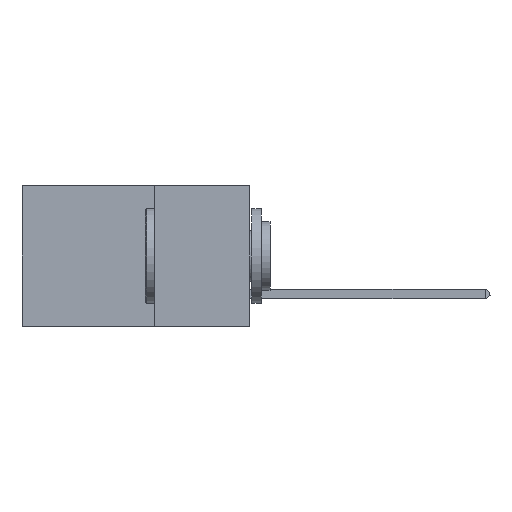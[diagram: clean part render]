
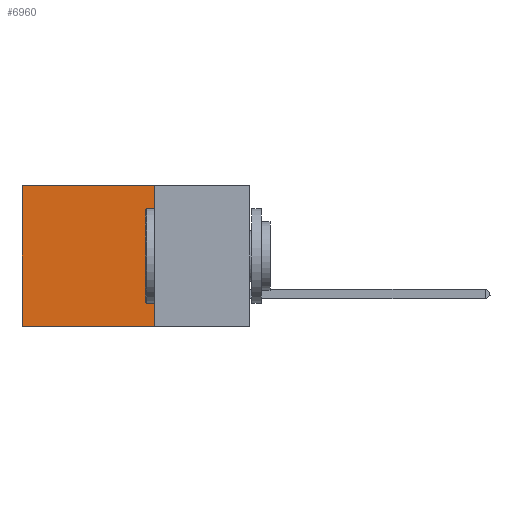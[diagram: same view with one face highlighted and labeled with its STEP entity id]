
A CAD part, left-side view. The second image highlights one B-rep face of the part: STEP entity #6960.
In plain terms, the highlighted planar face has unit normal (-1, 0, 0).
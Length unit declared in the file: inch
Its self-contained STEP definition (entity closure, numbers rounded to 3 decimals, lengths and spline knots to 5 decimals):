
#1176 = ORIENTED_EDGE ( 'NONE', *, *, #7756, .F. ) ;
#1188 = DIRECTION ( 'NONE',  ( 0., 0., -1. ) ) ;
#2180 = DIRECTION ( 'NONE',  ( 0., 1., 0. ) ) ;
#2406 = DIRECTION ( 'NONE',  ( 0., 0., -1. ) ) ;
#2745 = VECTOR ( 'NONE', #12073, 39.37008 ) ;
#2907 = CARTESIAN_POINT ( 'NONE',  ( 0.2875, 0.25, -0.37 ) ) ;
#2998 = VERTEX_POINT ( 'NONE', #14916 ) ;
#4323 = EDGE_CURVE ( 'NONE', #6081, #2998, #13148, .T. ) ;
#4479 = EDGE_CURVE ( 'NONE', #7516, #2998, #5208, .T. ) ;
#4719 = PLANE ( 'NONE',  #14520 ) ;
#4974 = CARTESIAN_POINT ( 'NONE',  ( 0.2875, 0.6, 0. ) ) ;
#5107 = CARTESIAN_POINT ( 'NONE',  ( 0.2875, 0.6, 0. ) ) ;
#5208 = LINE ( 'NONE', #2907, #2745 ) ;
#6081 = VERTEX_POINT ( 'NONE', #5107 ) ;
#6674 = VERTEX_POINT ( 'NONE', #11377 ) ;
#6960 = ADVANCED_FACE ( 'NONE', ( #15464 ), #4719, .F. ) ;
#7046 = VECTOR ( 'NONE', #2406, 39.37008 ) ;
#7516 = VERTEX_POINT ( 'NONE', #9724 ) ;
#7756 = EDGE_CURVE ( 'NONE', #6674, #7516, #9571, .T. ) ;
#8361 = VECTOR ( 'NONE', #16404, 39.37008 ) ;
#8381 = ORIENTED_EDGE ( 'NONE', *, *, #4479, .F. ) ;
#8797 = CARTESIAN_POINT ( 'NONE',  ( 0.2875, 0.25, 0. ) ) ;
#9001 = CARTESIAN_POINT ( 'NONE',  ( 0.2875, 0.25, 0. ) ) ;
#9236 = VECTOR ( 'NONE', #2180, 39.37008 ) ;
#9571 = LINE ( 'NONE', #8797, #8361 ) ;
#9724 = CARTESIAN_POINT ( 'NONE',  ( 0.2875, 0.25, -0.37 ) ) ;
#10005 = ORIENTED_EDGE ( 'NONE', *, *, #4323, .T. ) ;
#11377 = CARTESIAN_POINT ( 'NONE',  ( 0.2875, 0.25, 0. ) ) ;
#11438 = DIRECTION ( 'NONE',  ( 1., 0., 0. ) ) ;
#11677 = ORIENTED_EDGE ( 'NONE', *, *, #12270, .T. ) ;
#12073 = DIRECTION ( 'NONE',  ( 0., 1., 0. ) ) ;
#12266 = LINE ( 'NONE', #13863, #9236 ) ;
#12270 = EDGE_CURVE ( 'NONE', #6674, #6081, #12266, .T. ) ;
#13148 = LINE ( 'NONE', #4974, #7046 ) ;
#13863 = CARTESIAN_POINT ( 'NONE',  ( 0.2875, 0.25, 0. ) ) ;
#14520 = AXIS2_PLACEMENT_3D ( 'NONE', #9001, #11438, #1188 ) ;
#14916 = CARTESIAN_POINT ( 'NONE',  ( 0.2875, 0.6, -0.37 ) ) ;
#15464 = FACE_OUTER_BOUND ( 'NONE', #16457, .T. ) ;
#16404 = DIRECTION ( 'NONE',  ( 0., 0., -1. ) ) ;
#16457 = EDGE_LOOP ( 'NONE', ( #10005, #8381, #1176, #11677 ) ) ;
